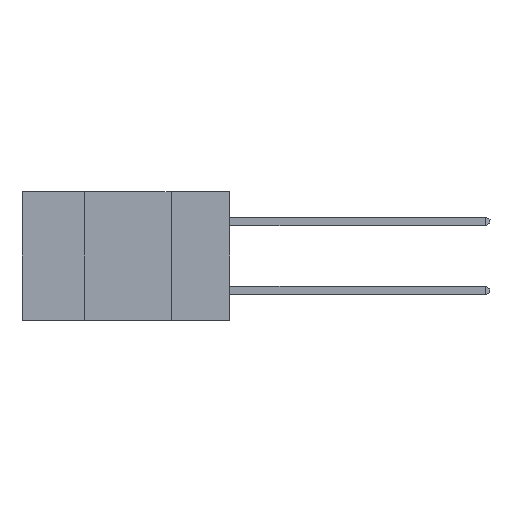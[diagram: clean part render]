
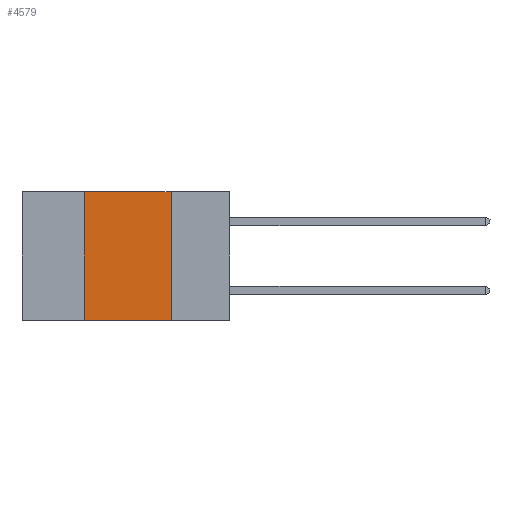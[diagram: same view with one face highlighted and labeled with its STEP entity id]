
A CAD part, left-side view. The second image highlights one B-rep face of the part: STEP entity #4579.
In plain terms, the highlighted planar face has unit normal (-1, 0, 0).
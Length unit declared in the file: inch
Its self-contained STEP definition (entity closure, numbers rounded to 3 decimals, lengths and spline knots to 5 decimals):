
#14 = LINE ( 'NONE', #4160, #8752 ) ;
#42 = CARTESIAN_POINT ( 'NONE',  ( 0., 0.42, -0.37 ) ) ;
#358 = AXIS2_PLACEMENT_3D ( 'NONE', #6874, #6922, #10061 ) ;
#600 = CARTESIAN_POINT ( 'NONE',  ( 0., 0.6, 0. ) ) ;
#1116 = EDGE_LOOP ( 'NONE', ( #10003, #9875, #7312, #7452 ) ) ;
#1177 = DIRECTION ( 'NONE',  ( 0., 0., -1. ) ) ;
#1365 = VERTEX_POINT ( 'NONE', #8194 ) ;
#1608 = VERTEX_POINT ( 'NONE', #7068 ) ;
#2154 = PLANE ( 'NONE',  #358 ) ;
#2407 = DIRECTION ( 'NONE',  ( 0., -1., 0. ) ) ;
#2828 = EDGE_CURVE ( 'NONE', #6324, #1365, #4777, .T. ) ;
#4130 = DIRECTION ( 'NONE',  ( 0., 0., 1. ) ) ;
#4160 = CARTESIAN_POINT ( 'NONE',  ( 0., 0.6, -0.37 ) ) ;
#4514 = EDGE_CURVE ( 'NONE', #1608, #6324, #8303, .T. ) ;
#4579 = ADVANCED_FACE ( 'NONE', ( #5214 ), #2154, .F. ) ;
#4777 = LINE ( 'NONE', #600, #9333 ) ;
#5214 = FACE_OUTER_BOUND ( 'NONE', #1116, .T. ) ;
#5257 = LINE ( 'NONE', #10202, #6082 ) ;
#6082 = VECTOR ( 'NONE', #1177, 39.37008 ) ;
#6324 = VERTEX_POINT ( 'NONE', #9578 ) ;
#6404 = VERTEX_POINT ( 'NONE', #9789 ) ;
#6785 = EDGE_CURVE ( 'NONE', #1608, #6404, #14, .T. ) ;
#6874 = CARTESIAN_POINT ( 'NONE',  ( 0., 0.6, 0. ) ) ;
#6922 = DIRECTION ( 'NONE',  ( 1., 0., 0. ) ) ;
#7068 = CARTESIAN_POINT ( 'NONE',  ( 0., 0.42, -0.37 ) ) ;
#7185 = VECTOR ( 'NONE', #4130, 39.37008 ) ;
#7312 = ORIENTED_EDGE ( 'NONE', *, *, #4514, .F. ) ;
#7452 = ORIENTED_EDGE ( 'NONE', *, *, #6785, .T. ) ;
#8194 = CARTESIAN_POINT ( 'NONE',  ( 0., 0.17, 0. ) ) ;
#8303 = LINE ( 'NONE', #42, #7185 ) ;
#8752 = VECTOR ( 'NONE', #2407, 39.37008 ) ;
#9333 = VECTOR ( 'NONE', #9468, 39.37008 ) ;
#9468 = DIRECTION ( 'NONE',  ( 0., -1., 0. ) ) ;
#9578 = CARTESIAN_POINT ( 'NONE',  ( 0., 0.42, 0. ) ) ;
#9789 = CARTESIAN_POINT ( 'NONE',  ( 0., 0.17, -0.37 ) ) ;
#9875 = ORIENTED_EDGE ( 'NONE', *, *, #2828, .F. ) ;
#10003 = ORIENTED_EDGE ( 'NONE', *, *, #10220, .F. ) ;
#10061 = DIRECTION ( 'NONE',  ( 0., 0., -1. ) ) ;
#10202 = CARTESIAN_POINT ( 'NONE',  ( 0., 0.17, -0.37 ) ) ;
#10220 = EDGE_CURVE ( 'NONE', #1365, #6404, #5257, .T. ) ;
